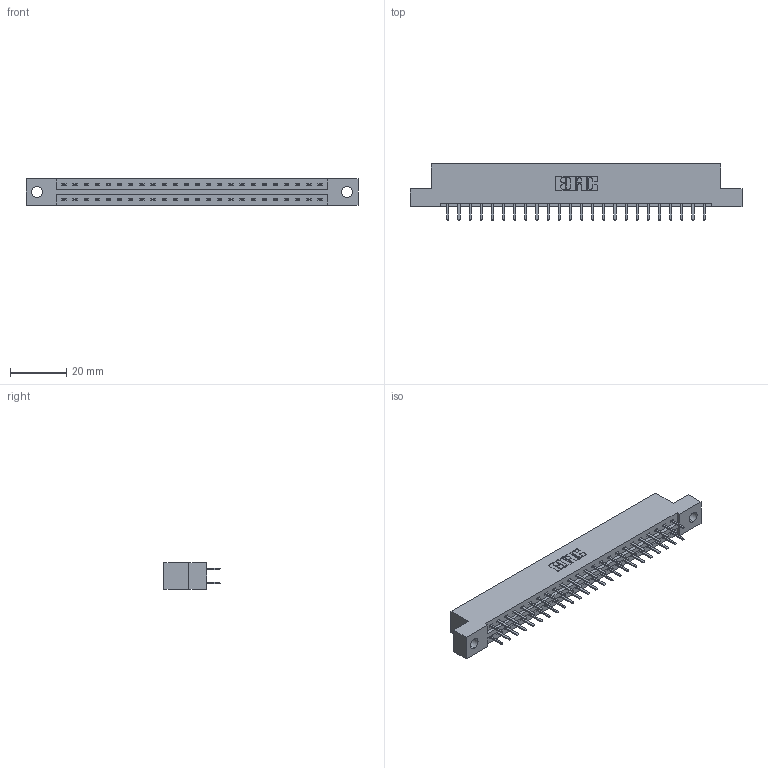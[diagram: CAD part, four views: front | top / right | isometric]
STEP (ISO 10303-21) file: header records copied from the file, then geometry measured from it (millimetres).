
FILE_DESCRIPTION (( 'STEP AP203' ), '1' );
FILE_NAME ('337-048-520-204.STEP', '2019-10-09T14:31:20', ( '' ), ( '' ), 'SwSTEP 2.0', 'SolidWorks 2016', '' );
FILE_SCHEMA (( 'CONFIG_CONTROL_DESIGN' ));
Length unit declared in the file: inch
Products named in the file (3): 337 Part_Flush Mounting Lugs - 0.156 Dia-TH; 337-048-520-204; 345-292-001_345-293-120
Assembly tree (49 placements, depth 2):
  337-048-520-204
    337 Part_Flush Mounting Lugs - 0.156 Dia-TH
    345-292-001_345-293-120  x48
Bounding box: 118.11 x 20.02 x 9.4 mm (x, y, z)
Volume: 12098.8 mm3; surface area: 13240.1 mm2
Topology: 49 solids, 49 shells, 2898 faces, 8423 edges, 5486 vertices
Faces by surface type: plane 1990, cylinder 908
Entity records: 21053 total; most frequent: CARTESIAN_POINT 3574, ORIENTED_EDGE 3498, DIRECTION 3061, EDGE_CURVE 1749, LINE 1617, VECTOR 1617, VERTEX_POINT 1162, AXIS2_PLACEMENT_3D 722
